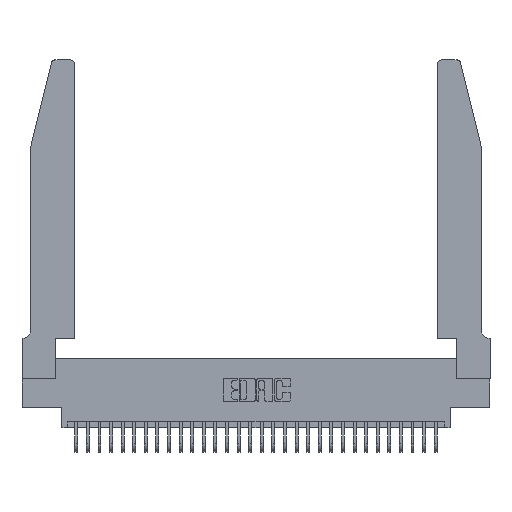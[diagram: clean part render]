
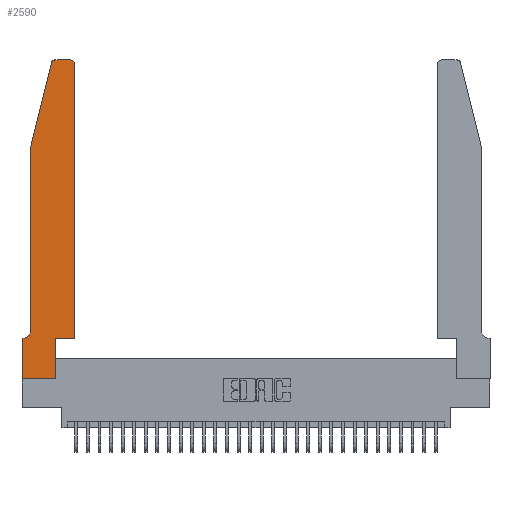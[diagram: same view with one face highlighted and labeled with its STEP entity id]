
A CAD part, top view. The second image highlights one B-rep face of the part: STEP entity #2590.
In plain terms, the highlighted planar face has unit normal (0, 0, 1).
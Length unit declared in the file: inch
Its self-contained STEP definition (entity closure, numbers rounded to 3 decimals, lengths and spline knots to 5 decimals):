
#242 = VERTEX_POINT ( 'NONE', #4466 ) ;
#304 = CARTESIAN_POINT ( 'NONE',  ( 0.4505, 0.35, 0.37 ) ) ;
#349 = VECTOR ( 'NONE', #9600, 39.37008 ) ;
#1497 = CARTESIAN_POINT ( 'NONE',  ( 0.284, 2.72, 0.37 ) ) ;
#1659 = VERTEX_POINT ( 'NONE', #25668 ) ;
#2524 = LINE ( 'NONE', #12887, #24051 ) ;
#2590 = ADVANCED_FACE ( 'NONE', ( #20001 ), #22733, .T. ) ;
#2742 = EDGE_CURVE ( 'NONE', #27042, #6653, #5620, .T. ) ;
#3042 = AXIS2_PLACEMENT_3D ( 'NONE', #9061, #24592, #29329 ) ;
#3453 = LINE ( 'NONE', #22267, #25753 ) ;
#3749 = DIRECTION ( 'NONE',  ( 1., 0., 0. ) ) ;
#4466 = CARTESIAN_POINT ( 'NONE',  ( 0.0055, 0.35, 0.37 ) ) ;
#5483 = CARTESIAN_POINT ( 'NONE',  ( 0.0755, 0.35, 0.37 ) ) ;
#5620 = LINE ( 'NONE', #20379, #21141 ) ;
#5745 = DIRECTION ( 'NONE',  ( 0., -1., 0. ) ) ;
#5998 = EDGE_CURVE ( 'NONE', #31046, #242, #17819, .T. ) ;
#6279 = VERTEX_POINT ( 'NONE', #19583 ) ;
#6355 = ORIENTED_EDGE ( 'NONE', *, *, #14621, .T. ) ;
#6514 = ORIENTED_EDGE ( 'NONE', *, *, #13590, .T. ) ;
#6653 = VERTEX_POINT ( 'NONE', #11837 ) ;
#6812 = EDGE_CURVE ( 'NONE', #242, #1659, #20933, .T. ) ;
#7135 = VERTEX_POINT ( 'NONE', #28453 ) ;
#7240 = VERTEX_POINT ( 'NONE', #10076 ) ;
#7374 = ORIENTED_EDGE ( 'NONE', *, *, #6812, .T. ) ;
#8084 = EDGE_CURVE ( 'NONE', #7240, #6279, #2524, .T. ) ;
#8369 = CIRCLE ( 'NONE', #3042, 0.03 ) ;
#8988 = ORIENTED_EDGE ( 'NONE', *, *, #30450, .T. ) ;
#9061 = CARTESIAN_POINT ( 'NONE',  ( 0.4205, 2.72, 0.37 ) ) ;
#9600 = DIRECTION ( 'NONE',  ( -1., 0., 0. ) ) ;
#9857 = CIRCLE ( 'NONE', #11877, 0.03 ) ;
#10076 = CARTESIAN_POINT ( 'NONE',  ( 0., 0., 0.37 ) ) ;
#10768 = CARTESIAN_POINT ( 'NONE',  ( 0.284, 2.75, 0.37 ) ) ;
#11292 = ORIENTED_EDGE ( 'NONE', *, *, #2742, .T. ) ;
#11837 = CARTESIAN_POINT ( 'NONE',  ( 0.4505, 2.72, 0.37 ) ) ;
#11877 = AXIS2_PLACEMENT_3D ( 'NONE', #1497, #31855, #14165 ) ;
#12521 = CARTESIAN_POINT ( 'NONE',  ( 0.0755, 2., 0.37 ) ) ;
#12651 = ORIENTED_EDGE ( 'NONE', *, *, #26122, .T. ) ;
#12695 = DIRECTION ( 'NONE',  ( -1., 0., 0. ) ) ;
#12842 = EDGE_CURVE ( 'NONE', #29858, #19165, #21520, .T. ) ;
#12887 = CARTESIAN_POINT ( 'NONE',  ( 0., 0., 0.37 ) ) ;
#13590 = EDGE_CURVE ( 'NONE', #6653, #29858, #8369, .T. ) ;
#13814 = DIRECTION ( 'NONE',  ( 0., 1., 0. ) ) ;
#14102 = ORIENTED_EDGE ( 'NONE', *, *, #8084, .T. ) ;
#14165 = DIRECTION ( 'NONE',  ( 1., 0., 0. ) ) ;
#14528 = CARTESIAN_POINT ( 'NONE',  ( 0.2605, 2.75, 0.37 ) ) ;
#14621 = EDGE_CURVE ( 'NONE', #1659, #7240, #3453, .T. ) ;
#14848 = AXIS2_PLACEMENT_3D ( 'NONE', #19951, #25059, #20176 ) ;
#15528 = DIRECTION ( 'NONE',  ( 0., 1., 0. ) ) ;
#16267 = CARTESIAN_POINT ( 'NONE',  ( 0.0755, 2., 0.37 ) ) ;
#16399 = CARTESIAN_POINT ( 'NONE',  ( 0.25487, 2.72718, 0.37 ) ) ;
#17819 = CIRCLE ( 'NONE', #23975, 0.07 ) ;
#18204 = VERTEX_POINT ( 'NONE', #32424 ) ;
#18479 = ORIENTED_EDGE ( 'NONE', *, *, #5998, .T. ) ;
#19165 = VERTEX_POINT ( 'NONE', #10768 ) ;
#19255 = LINE ( 'NONE', #16267, #25224 ) ;
#19583 = CARTESIAN_POINT ( 'NONE',  ( 0.2865, 0., 0.37 ) ) ;
#19951 = CARTESIAN_POINT ( 'NONE',  ( 0., 0.35, 0.37 ) ) ;
#20001 = FACE_OUTER_BOUND ( 'NONE', #22742, .T. ) ;
#20176 = DIRECTION ( 'NONE',  ( 1., 0., 0. ) ) ;
#20202 = VECTOR ( 'NONE', #13814, 39.37008 ) ;
#20379 = CARTESIAN_POINT ( 'NONE',  ( 0.4505, 0.35, 0.37 ) ) ;
#20933 = LINE ( 'NONE', #5483, #28471 ) ;
#21141 = VECTOR ( 'NONE', #15528, 39.37008 ) ;
#21413 = CARTESIAN_POINT ( 'NONE',  ( 0.2865, 0.35, 0.37 ) ) ;
#21520 = LINE ( 'NONE', #14528, #349 ) ;
#22267 = CARTESIAN_POINT ( 'NONE',  ( 0., 0., 0.37 ) ) ;
#22733 = PLANE ( 'NONE',  #14848 ) ;
#22742 = EDGE_LOOP ( 'NONE', ( #31412, #29706, #25771, #12651, #18479, #7374, #6355, #14102, #8988, #32534, #11292, #6514 ) ) ;
#23289 = VECTOR ( 'NONE', #3749, 39.37008 ) ;
#23975 = AXIS2_PLACEMENT_3D ( 'NONE', #29642, #32212, #12695 ) ;
#24051 = VECTOR ( 'NONE', #30580, 39.37008 ) ;
#24592 = DIRECTION ( 'NONE',  ( 0., 0., 1. ) ) ;
#25059 = DIRECTION ( 'NONE',  ( 0., 0., 1. ) ) ;
#25224 = VECTOR ( 'NONE', #26526, 39.37008 ) ;
#25428 = DIRECTION ( 'NONE',  ( -1., 0., 0. ) ) ;
#25668 = CARTESIAN_POINT ( 'NONE',  ( 0., 0.35, 0.37 ) ) ;
#25753 = VECTOR ( 'NONE', #5745, 39.37008 ) ;
#25771 = ORIENTED_EDGE ( 'NONE', *, *, #26609, .T. ) ;
#25994 = LINE ( 'NONE', #12521, #29982 ) ;
#26037 = LINE ( 'NONE', #26329, #23289 ) ;
#26122 = EDGE_CURVE ( 'NONE', #18204, #31046, #25994, .T. ) ;
#26154 = CARTESIAN_POINT ( 'NONE',  ( 0.0755, 0.42, 0.37 ) ) ;
#26329 = CARTESIAN_POINT ( 'NONE',  ( 0.4505, 0.35, 0.37 ) ) ;
#26526 = DIRECTION ( 'NONE',  ( -0.239, -0.971, 0. ) ) ;
#26609 = EDGE_CURVE ( 'NONE', #31800, #18204, #19255, .T. ) ;
#27042 = VERTEX_POINT ( 'NONE', #304 ) ;
#28120 = LINE ( 'NONE', #21413, #20202 ) ;
#28453 = CARTESIAN_POINT ( 'NONE',  ( 0.2865, 0.35, 0.37 ) ) ;
#28471 = VECTOR ( 'NONE', #25428, 39.37008 ) ;
#29329 = DIRECTION ( 'NONE',  ( 1., 0., 0. ) ) ;
#29642 = CARTESIAN_POINT ( 'NONE',  ( 0.0055, 0.42, 0.37 ) ) ;
#29706 = ORIENTED_EDGE ( 'NONE', *, *, #30631, .T. ) ;
#29858 = VERTEX_POINT ( 'NONE', #30699 ) ;
#29982 = VECTOR ( 'NONE', #30018, 39.37008 ) ;
#30018 = DIRECTION ( 'NONE',  ( 0., -1., 0. ) ) ;
#30450 = EDGE_CURVE ( 'NONE', #6279, #7135, #28120, .T. ) ;
#30580 = DIRECTION ( 'NONE',  ( 1., 0., 0. ) ) ;
#30631 = EDGE_CURVE ( 'NONE', #19165, #31800, #9857, .T. ) ;
#30699 = CARTESIAN_POINT ( 'NONE',  ( 0.4205, 2.75, 0.37 ) ) ;
#31046 = VERTEX_POINT ( 'NONE', #26154 ) ;
#31412 = ORIENTED_EDGE ( 'NONE', *, *, #12842, .T. ) ;
#31800 = VERTEX_POINT ( 'NONE', #16399 ) ;
#31814 = EDGE_CURVE ( 'NONE', #7135, #27042, #26037, .T. ) ;
#31855 = DIRECTION ( 'NONE',  ( 0., 0., 1. ) ) ;
#32212 = DIRECTION ( 'NONE',  ( 0., 0., -1. ) ) ;
#32424 = CARTESIAN_POINT ( 'NONE',  ( 0.0755, 2., 0.37 ) ) ;
#32534 = ORIENTED_EDGE ( 'NONE', *, *, #31814, .T. ) ;
